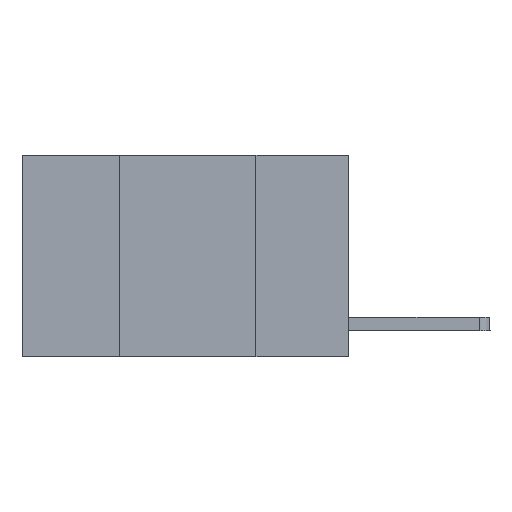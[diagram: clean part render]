
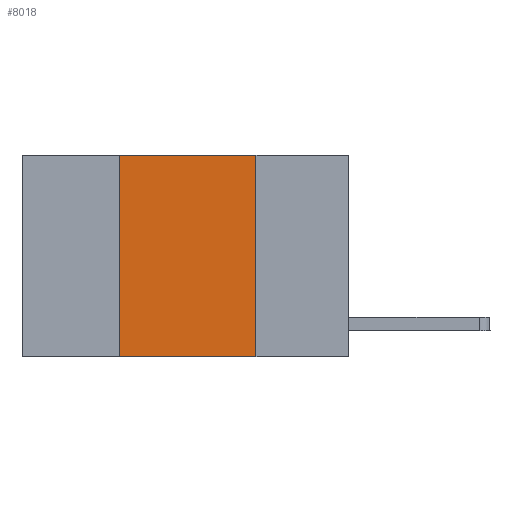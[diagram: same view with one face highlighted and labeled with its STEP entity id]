
A CAD part, left-side view. The second image highlights one B-rep face of the part: STEP entity #8018.
In plain terms, the highlighted planar face has unit normal (-1, 0, 0).
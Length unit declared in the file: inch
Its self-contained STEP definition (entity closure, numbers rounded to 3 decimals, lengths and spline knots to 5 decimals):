
#435 = EDGE_CURVE ( 'NONE', #1246, #8918, #7245, .T. ) ;
#928 = DIRECTION ( 'NONE',  ( 0., 0., -1. ) ) ;
#1011 = DIRECTION ( 'NONE',  ( 0., 0., -1. ) ) ;
#1246 = VERTEX_POINT ( 'NONE', #10477 ) ;
#1281 = LINE ( 'NONE', #8012, #6729 ) ;
#1521 = AXIS2_PLACEMENT_3D ( 'NONE', #3580, #5309, #1011 ) ;
#1621 = ORIENTED_EDGE ( 'NONE', *, *, #10419, .F. ) ;
#1887 = FACE_OUTER_BOUND ( 'NONE', #2121, .T. ) ;
#2082 = CARTESIAN_POINT ( 'NONE',  ( 0., 0.6, 0. ) ) ;
#2121 = EDGE_LOOP ( 'NONE', ( #6611, #1621, #4857, #2707 ) ) ;
#2332 = DIRECTION ( 'NONE',  ( 0., 0., 1. ) ) ;
#2707 = ORIENTED_EDGE ( 'NONE', *, *, #9956, .T. ) ;
#2962 = CARTESIAN_POINT ( 'NONE',  ( 0., 0.17, -0.37 ) ) ;
#3000 = VERTEX_POINT ( 'NONE', #4104 ) ;
#3580 = CARTESIAN_POINT ( 'NONE',  ( 0., 0.6, 0. ) ) ;
#3965 = VECTOR ( 'NONE', #928, 39.37008 ) ;
#4104 = CARTESIAN_POINT ( 'NONE',  ( 0., 0.17, 0. ) ) ;
#4723 = DIRECTION ( 'NONE',  ( 0., -1., 0. ) ) ;
#4857 = ORIENTED_EDGE ( 'NONE', *, *, #435, .F. ) ;
#5309 = DIRECTION ( 'NONE',  ( 1., 0., 0. ) ) ;
#5464 = DIRECTION ( 'NONE',  ( 0., -1., 0. ) ) ;
#6035 = CARTESIAN_POINT ( 'NONE',  ( 0., 0.42, 0. ) ) ;
#6250 = LINE ( 'NONE', #2082, #6737 ) ;
#6611 = ORIENTED_EDGE ( 'NONE', *, *, #10266, .F. ) ;
#6729 = VECTOR ( 'NONE', #4723, 39.37008 ) ;
#6737 = VECTOR ( 'NONE', #5464, 39.37008 ) ;
#6783 = VECTOR ( 'NONE', #2332, 39.37008 ) ;
#6837 = PLANE ( 'NONE',  #1521 ) ;
#7245 = LINE ( 'NONE', #9837, #6783 ) ;
#8012 = CARTESIAN_POINT ( 'NONE',  ( 0., 0.6, -0.37 ) ) ;
#8018 = ADVANCED_FACE ( 'NONE', ( #1887 ), #6837, .F. ) ;
#8423 = CARTESIAN_POINT ( 'NONE',  ( 0., 0.17, 0. ) ) ;
#8918 = VERTEX_POINT ( 'NONE', #6035 ) ;
#9117 = VERTEX_POINT ( 'NONE', #2962 ) ;
#9837 = CARTESIAN_POINT ( 'NONE',  ( 0., 0.42, 0. ) ) ;
#9956 = EDGE_CURVE ( 'NONE', #1246, #9117, #1281, .T. ) ;
#10266 = EDGE_CURVE ( 'NONE', #3000, #9117, #10290, .T. ) ;
#10290 = LINE ( 'NONE', #8423, #3965 ) ;
#10419 = EDGE_CURVE ( 'NONE', #8918, #3000, #6250, .T. ) ;
#10477 = CARTESIAN_POINT ( 'NONE',  ( 0., 0.42, -0.37 ) ) ;
